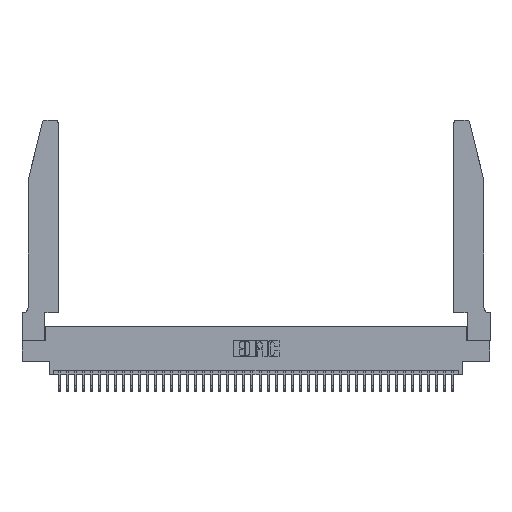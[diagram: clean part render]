
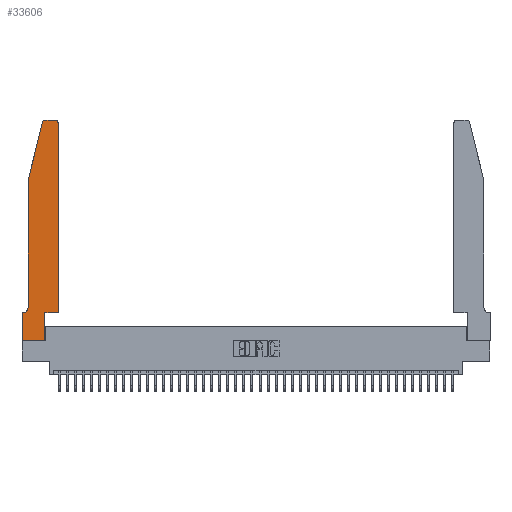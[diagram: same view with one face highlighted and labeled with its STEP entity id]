
A CAD part, top view. The second image highlights one B-rep face of the part: STEP entity #33606.
In plain terms, the highlighted planar face has unit normal (0, 0, 1).
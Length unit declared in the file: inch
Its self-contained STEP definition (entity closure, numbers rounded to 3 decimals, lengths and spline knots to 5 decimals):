
#217 = DIRECTION ( 'NONE',  ( -1., 0., 0. ) ) ;
#431 = ORIENTED_EDGE ( 'NONE', *, *, #34730, .T. ) ;
#636 = VECTOR ( 'NONE', #19717, 39.37008 ) ;
#1037 = CIRCLE ( 'NONE', #38275, 0.03 ) ;
#1159 = CARTESIAN_POINT ( 'NONE',  ( 0.4505, 2.72, 0.37 ) ) ;
#1160 = DIRECTION ( 'NONE',  ( 0., 1., 0. ) ) ;
#1200 = VERTEX_POINT ( 'NONE', #40863 ) ;
#1521 = CARTESIAN_POINT ( 'NONE',  ( 0.2865, 0., 0.37 ) ) ;
#1534 = CARTESIAN_POINT ( 'NONE',  ( 0.4505, 0.35, 0.37 ) ) ;
#2387 = VERTEX_POINT ( 'NONE', #13725 ) ;
#2998 = VERTEX_POINT ( 'NONE', #27291 ) ;
#3252 = VECTOR ( 'NONE', #26408, 39.37008 ) ;
#3366 = ORIENTED_EDGE ( 'NONE', *, *, #39434, .T. ) ;
#3476 = ORIENTED_EDGE ( 'NONE', *, *, #24150, .T. ) ;
#4183 = CARTESIAN_POINT ( 'NONE',  ( 0., 0., 0.37 ) ) ;
#4630 = CARTESIAN_POINT ( 'NONE',  ( 0.2865, 0.35, 0.37 ) ) ;
#4980 = DIRECTION ( 'NONE',  ( 0., 1., 0. ) ) ;
#5150 = VERTEX_POINT ( 'NONE', #13261 ) ;
#5416 = DIRECTION ( 'NONE',  ( 0., 0., 1. ) ) ;
#5702 = CARTESIAN_POINT ( 'NONE',  ( 0.0755, 2., 0.37 ) ) ;
#5902 = DIRECTION ( 'NONE',  ( 0., 0., 1. ) ) ;
#6194 = LINE ( 'NONE', #35470, #23479 ) ;
#6415 = DIRECTION ( 'NONE',  ( 0., 0., -1. ) ) ;
#6621 = ORIENTED_EDGE ( 'NONE', *, *, #25277, .T. ) ;
#7157 = AXIS2_PLACEMENT_3D ( 'NONE', #26124, #5416, #29605 ) ;
#7960 = AXIS2_PLACEMENT_3D ( 'NONE', #12302, #15768, #39960 ) ;
#8028 = EDGE_CURVE ( 'NONE', #1200, #2998, #37858, .T. ) ;
#8462 = ORIENTED_EDGE ( 'NONE', *, *, #19051, .T. ) ;
#8806 = PLANE ( 'NONE',  #7960 ) ;
#9439 = EDGE_CURVE ( 'NONE', #5150, #2387, #34520, .T. ) ;
#10480 = EDGE_CURVE ( 'NONE', #32511, #5150, #42704, .T. ) ;
#11010 = CARTESIAN_POINT ( 'NONE',  ( 0.2865, 0.35, 0.37 ) ) ;
#11168 = VERTEX_POINT ( 'NONE', #11010 ) ;
#11680 = DIRECTION ( 'NONE',  ( 0., -1., 0. ) ) ;
#12302 = CARTESIAN_POINT ( 'NONE',  ( 0., 0.35, 0.37 ) ) ;
#12515 = VECTOR ( 'NONE', #4980, 39.37008 ) ;
#13261 = CARTESIAN_POINT ( 'NONE',  ( 0.0055, 0.35, 0.37 ) ) ;
#13725 = CARTESIAN_POINT ( 'NONE',  ( 0., 0.35, 0.37 ) ) ;
#13835 = VECTOR ( 'NONE', #1160, 39.37008 ) ;
#13879 = VERTEX_POINT ( 'NONE', #37300 ) ;
#14875 = VECTOR ( 'NONE', #217, 39.37008 ) ;
#14973 = ORIENTED_EDGE ( 'NONE', *, *, #8028, .T. ) ;
#15021 = ORIENTED_EDGE ( 'NONE', *, *, #9439, .T. ) ;
#15768 = DIRECTION ( 'NONE',  ( 0., 0., 1. ) ) ;
#17019 = AXIS2_PLACEMENT_3D ( 'NONE', #27115, #6415, #30595 ) ;
#17906 = CARTESIAN_POINT ( 'NONE',  ( 0., 0., 0.37 ) ) ;
#18218 = ORIENTED_EDGE ( 'NONE', *, *, #10480, .T. ) ;
#18260 = ORIENTED_EDGE ( 'NONE', *, *, #20812, .T. ) ;
#18585 = EDGE_CURVE ( 'NONE', #32770, #11168, #23026, .T. ) ;
#19051 = EDGE_CURVE ( 'NONE', #13879, #31569, #24070, .T. ) ;
#19717 = DIRECTION ( 'NONE',  ( 0., -1., 0. ) ) ;
#20812 = EDGE_CURVE ( 'NONE', #2387, #23236, #37415, .T. ) ;
#22118 = VERTEX_POINT ( 'NONE', #42615 ) ;
#22616 = ORIENTED_EDGE ( 'NONE', *, *, #18585, .T. ) ;
#23026 = LINE ( 'NONE', #4630, #13835 ) ;
#23236 = VERTEX_POINT ( 'NONE', #17906 ) ;
#23479 = VECTOR ( 'NONE', #38924, 39.37008 ) ;
#24070 = LINE ( 'NONE', #41626, #14875 ) ;
#24150 = EDGE_CURVE ( 'NONE', #22118, #34804, #30917, .T. ) ;
#24215 = VECTOR ( 'NONE', #24323, 39.37008 ) ;
#24314 = CIRCLE ( 'NONE', #7157, 0.03 ) ;
#24323 = DIRECTION ( 'NONE',  ( -1., 0., 0. ) ) ;
#25277 = EDGE_CURVE ( 'NONE', #34804, #13879, #24314, .T. ) ;
#26124 = CARTESIAN_POINT ( 'NONE',  ( 0.4205, 2.72, 0.37 ) ) ;
#26408 = DIRECTION ( 'NONE',  ( -0.239, -0.971, 0. ) ) ;
#26606 = CARTESIAN_POINT ( 'NONE',  ( 0.284, 2.72, 0.37 ) ) ;
#27115 = CARTESIAN_POINT ( 'NONE',  ( 0.0055, 0.42, 0.37 ) ) ;
#27291 = CARTESIAN_POINT ( 'NONE',  ( 0.0755, 2., 0.37 ) ) ;
#28128 = EDGE_CURVE ( 'NONE', #2998, #32511, #42434, .T. ) ;
#29251 = EDGE_LOOP ( 'NONE', ( #8462, #39304, #14973, #44676, #18218, #15021, #18260, #431, #22616, #3366, #3476, #6621 ) ) ;
#29522 = VECTOR ( 'NONE', #38656, 39.37008 ) ;
#29605 = DIRECTION ( 'NONE',  ( 1., 0., 0. ) ) ;
#30083 = DIRECTION ( 'NONE',  ( 1., 0., 0. ) ) ;
#30595 = DIRECTION ( 'NONE',  ( -1., 0., 0. ) ) ;
#30917 = LINE ( 'NONE', #1534, #12515 ) ;
#31132 = CARTESIAN_POINT ( 'NONE',  ( 0.0755, 0.35, 0.37 ) ) ;
#31569 = VERTEX_POINT ( 'NONE', #33524 ) ;
#32511 = VERTEX_POINT ( 'NONE', #38253 ) ;
#32770 = VERTEX_POINT ( 'NONE', #1521 ) ;
#33524 = CARTESIAN_POINT ( 'NONE',  ( 0.284, 2.75, 0.37 ) ) ;
#33606 = ADVANCED_FACE ( 'NONE', ( #38850 ), #8806, .T. ) ;
#34520 = LINE ( 'NONE', #31132, #24215 ) ;
#34730 = EDGE_CURVE ( 'NONE', #23236, #32770, #38719, .T. ) ;
#34804 = VERTEX_POINT ( 'NONE', #1159 ) ;
#35470 = CARTESIAN_POINT ( 'NONE',  ( 0.4505, 0.35, 0.37 ) ) ;
#37300 = CARTESIAN_POINT ( 'NONE',  ( 0.4205, 2.75, 0.37 ) ) ;
#37415 = LINE ( 'NONE', #40280, #636 ) ;
#37858 = LINE ( 'NONE', #5702, #3252 ) ;
#38253 = CARTESIAN_POINT ( 'NONE',  ( 0.0755, 0.42, 0.37 ) ) ;
#38275 = AXIS2_PLACEMENT_3D ( 'NONE', #26606, #5902, #30083 ) ;
#38656 = DIRECTION ( 'NONE',  ( 1., 0., 0. ) ) ;
#38719 = LINE ( 'NONE', #4183, #29522 ) ;
#38850 = FACE_OUTER_BOUND ( 'NONE', #29251, .T. ) ;
#38924 = DIRECTION ( 'NONE',  ( 1., 0., 0. ) ) ;
#39304 = ORIENTED_EDGE ( 'NONE', *, *, #42147, .T. ) ;
#39348 = CARTESIAN_POINT ( 'NONE',  ( 0.0755, 2., 0.37 ) ) ;
#39434 = EDGE_CURVE ( 'NONE', #11168, #22118, #6194, .T. ) ;
#39960 = DIRECTION ( 'NONE',  ( 1., 0., 0. ) ) ;
#40280 = CARTESIAN_POINT ( 'NONE',  ( 0., 0., 0.37 ) ) ;
#40863 = CARTESIAN_POINT ( 'NONE',  ( 0.25487, 2.72718, 0.37 ) ) ;
#41347 = VECTOR ( 'NONE', #11680, 39.37008 ) ;
#41626 = CARTESIAN_POINT ( 'NONE',  ( 0.2605, 2.75, 0.37 ) ) ;
#42147 = EDGE_CURVE ( 'NONE', #31569, #1200, #1037, .T. ) ;
#42434 = LINE ( 'NONE', #39348, #41347 ) ;
#42615 = CARTESIAN_POINT ( 'NONE',  ( 0.4505, 0.35, 0.37 ) ) ;
#42704 = CIRCLE ( 'NONE', #17019, 0.07 ) ;
#44676 = ORIENTED_EDGE ( 'NONE', *, *, #28128, .T. ) ;
